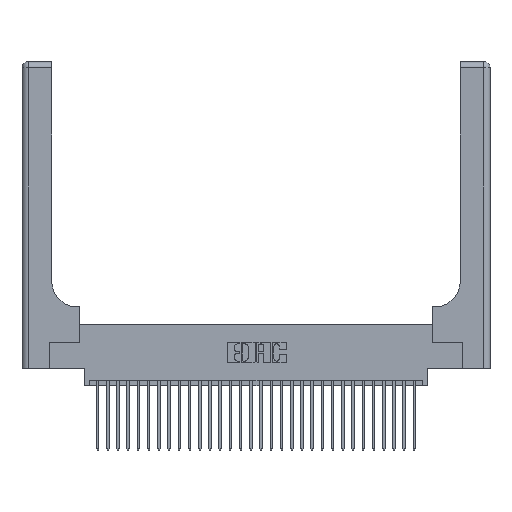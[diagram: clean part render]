
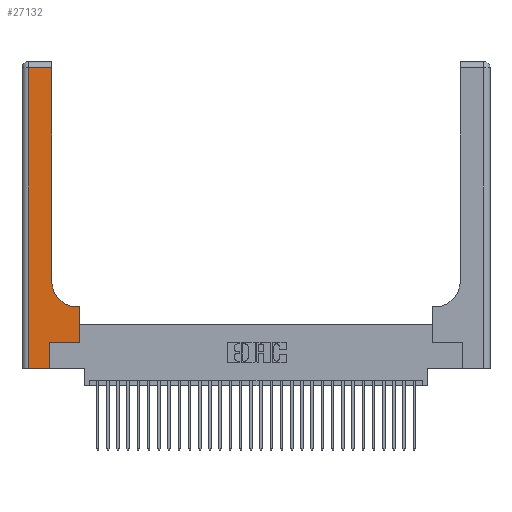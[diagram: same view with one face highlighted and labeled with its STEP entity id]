
A CAD part, top view. The second image highlights one B-rep face of the part: STEP entity #27132.
In plain terms, the highlighted planar face has unit normal (0, 0, 1).
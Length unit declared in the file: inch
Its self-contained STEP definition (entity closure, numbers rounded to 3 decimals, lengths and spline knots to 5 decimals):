
#340 = EDGE_CURVE ( 'NONE', #23236, #12850, #27070, .T. ) ;
#516 = EDGE_CURVE ( 'NONE', #8397, #29778, #9540, .T. ) ;
#1104 = CARTESIAN_POINT ( 'NONE',  ( 0.269, 0., 0.37 ) ) ;
#2035 = VECTOR ( 'NONE', #26418, 39.37008 ) ;
#2215 = LINE ( 'NONE', #9618, #15460 ) ;
#2328 = ORIENTED_EDGE ( 'NONE', *, *, #18485, .T. ) ;
#2346 = DIRECTION ( 'NONE',  ( 0., 0., -1. ) ) ;
#4076 = CARTESIAN_POINT ( 'NONE',  ( 0., 2.94, 0.37 ) ) ;
#5648 = EDGE_CURVE ( 'NONE', #12850, #8485, #31564, .T. ) ;
#6378 = EDGE_CURVE ( 'NONE', #16395, #28490, #30385, .T. ) ;
#6384 = CARTESIAN_POINT ( 'NONE',  ( 0.06, 3., 0.37 ) ) ;
#6618 = DIRECTION ( 'NONE',  ( -1., 0., 0. ) ) ;
#8123 = ORIENTED_EDGE ( 'NONE', *, *, #21572, .T. ) ;
#8397 = VERTEX_POINT ( 'NONE', #19838 ) ;
#8485 = VERTEX_POINT ( 'NONE', #27439 ) ;
#8767 = VECTOR ( 'NONE', #9302, 39.37008 ) ;
#9302 = DIRECTION ( 'NONE',  ( 0., 1., 0. ) ) ;
#9424 = AXIS2_PLACEMENT_3D ( 'NONE', #13604, #30537, #16049 ) ;
#9540 = LINE ( 'NONE', #23948, #8767 ) ;
#9618 = CARTESIAN_POINT ( 'NONE',  ( 0.2915, 0.6, 0.37 ) ) ;
#10435 = VECTOR ( 'NONE', #16029, 39.37008 ) ;
#11011 = CARTESIAN_POINT ( 'NONE',  ( 0.269, 0.25, 0.37 ) ) ;
#11252 = LINE ( 'NONE', #4076, #23478 ) ;
#12110 = DIRECTION ( 'NONE',  ( -1., 0., 0. ) ) ;
#12303 = EDGE_CURVE ( 'NONE', #28490, #17031, #16271, .T. ) ;
#12850 = VERTEX_POINT ( 'NONE', #14613 ) ;
#13604 = CARTESIAN_POINT ( 'NONE',  ( 0.5415, 0.85, 0.37 ) ) ;
#14227 = ORIENTED_EDGE ( 'NONE', *, *, #12303, .T. ) ;
#14391 = ORIENTED_EDGE ( 'NONE', *, *, #340, .T. ) ;
#14445 = ORIENTED_EDGE ( 'NONE', *, *, #516, .T. ) ;
#14613 = CARTESIAN_POINT ( 'NONE',  ( 0.2915, 0.85, 0.37 ) ) ;
#15284 = LINE ( 'NONE', #24040, #2035 ) ;
#15460 = VECTOR ( 'NONE', #12110, 39.37008 ) ;
#16029 = DIRECTION ( 'NONE',  ( 0., 1., 0. ) ) ;
#16049 = DIRECTION ( 'NONE',  ( 1., 0., 0. ) ) ;
#16271 = LINE ( 'NONE', #26119, #28377 ) ;
#16395 = VERTEX_POINT ( 'NONE', #19698 ) ;
#16870 = EDGE_LOOP ( 'NONE', ( #18967, #8123, #25711, #14227, #2328, #19152, #14445, #23175, #14391 ) ) ;
#16925 = EDGE_CURVE ( 'NONE', #29778, #23236, #2215, .T. ) ;
#17031 = VERTEX_POINT ( 'NONE', #17307 ) ;
#17221 = PLANE ( 'NONE',  #25014 ) ;
#17307 = CARTESIAN_POINT ( 'NONE',  ( 0.269, 0., 0.37 ) ) ;
#17532 = VECTOR ( 'NONE', #18611, 39.37008 ) ;
#17659 = CARTESIAN_POINT ( 'NONE',  ( 0.06, 0., 0.37 ) ) ;
#18485 = EDGE_CURVE ( 'NONE', #17031, #29224, #24210, .T. ) ;
#18611 = DIRECTION ( 'NONE',  ( 0., -1., 0. ) ) ;
#18967 = ORIENTED_EDGE ( 'NONE', *, *, #5648, .T. ) ;
#19152 = ORIENTED_EDGE ( 'NONE', *, *, #20404, .T. ) ;
#19689 = DIRECTION ( 'NONE',  ( -1., 0., 0. ) ) ;
#19698 = CARTESIAN_POINT ( 'NONE',  ( 0.06, 2.94, 0.37 ) ) ;
#19838 = CARTESIAN_POINT ( 'NONE',  ( 0.5585, 0.25, 0.37 ) ) ;
#20404 = EDGE_CURVE ( 'NONE', #29224, #8397, #15284, .T. ) ;
#21572 = EDGE_CURVE ( 'NONE', #8485, #16395, #11252, .T. ) ;
#22799 = CARTESIAN_POINT ( 'NONE',  ( 0.2915, 3., 0.37 ) ) ;
#23175 = ORIENTED_EDGE ( 'NONE', *, *, #16925, .T. ) ;
#23236 = VERTEX_POINT ( 'NONE', #30550 ) ;
#23478 = VECTOR ( 'NONE', #6618, 39.37008 ) ;
#23713 = VECTOR ( 'NONE', #29926, 39.37008 ) ;
#23948 = CARTESIAN_POINT ( 'NONE',  ( 0.5585, 0.25, 0.37 ) ) ;
#24040 = CARTESIAN_POINT ( 'NONE',  ( 0.269, 0.25, 0.37 ) ) ;
#24210 = LINE ( 'NONE', #1104, #10435 ) ;
#25014 = AXIS2_PLACEMENT_3D ( 'NONE', #29275, #2346, #19689 ) ;
#25711 = ORIENTED_EDGE ( 'NONE', *, *, #6378, .T. ) ;
#26119 = CARTESIAN_POINT ( 'NONE',  ( 0., 0., 0.37 ) ) ;
#26418 = DIRECTION ( 'NONE',  ( 1., 0., 0. ) ) ;
#27070 = CIRCLE ( 'NONE', #9424, 0.25 ) ;
#27132 = ADVANCED_FACE ( 'NONE', ( #28389 ), #17221, .F. ) ;
#27439 = CARTESIAN_POINT ( 'NONE',  ( 0.2915, 2.94, 0.37 ) ) ;
#27949 = CARTESIAN_POINT ( 'NONE',  ( 0.5585, 0.6, 0.37 ) ) ;
#28377 = VECTOR ( 'NONE', #28414, 39.37008 ) ;
#28389 = FACE_OUTER_BOUND ( 'NONE', #16870, .T. ) ;
#28414 = DIRECTION ( 'NONE',  ( 1., 0., 0. ) ) ;
#28490 = VERTEX_POINT ( 'NONE', #17659 ) ;
#29224 = VERTEX_POINT ( 'NONE', #11011 ) ;
#29275 = CARTESIAN_POINT ( 'NONE',  ( 0., 3., 0.37 ) ) ;
#29778 = VERTEX_POINT ( 'NONE', #27949 ) ;
#29926 = DIRECTION ( 'NONE',  ( 0., 1., 0. ) ) ;
#30385 = LINE ( 'NONE', #6384, #17532 ) ;
#30537 = DIRECTION ( 'NONE',  ( 0., 0., -1. ) ) ;
#30550 = CARTESIAN_POINT ( 'NONE',  ( 0.5415, 0.6, 0.37 ) ) ;
#31564 = LINE ( 'NONE', #22799, #23713 ) ;
